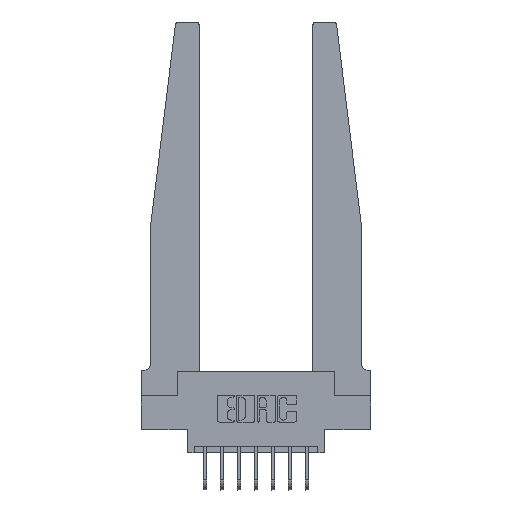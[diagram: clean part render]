
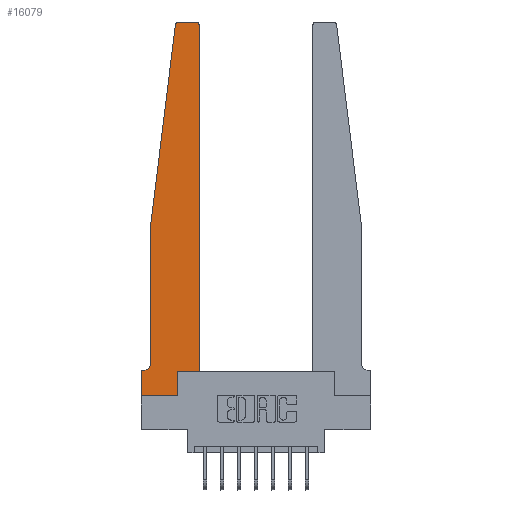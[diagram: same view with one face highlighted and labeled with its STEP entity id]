
A CAD part, top view. The second image highlights one B-rep face of the part: STEP entity #16079.
In plain terms, the highlighted planar face has unit normal (0, 0, 1).
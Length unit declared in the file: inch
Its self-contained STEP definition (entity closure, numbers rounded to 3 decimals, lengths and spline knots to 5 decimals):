
#207 = DIRECTION ( 'NONE',  ( -1., 0., 0. ) ) ;
#374 = ORIENTED_EDGE ( 'NONE', *, *, #4629, .T. ) ;
#394 = CARTESIAN_POINT ( 'NONE',  ( 0.425, 2.72, 0.37 ) ) ;
#516 = VECTOR ( 'NONE', #6131, 39.37008 ) ;
#575 = DIRECTION ( 'NONE',  ( 0., 0., 1. ) ) ;
#1018 = AXIS2_PLACEMENT_3D ( 'NONE', #13796, #10324, #2430 ) ;
#1557 = CARTESIAN_POINT ( 'NONE',  ( 0.425, 0.18, 0.37 ) ) ;
#1692 = EDGE_LOOP ( 'NONE', ( #10628, #9518, #12630, #6808, #10252, #374, #15915, #11730, #1996, #14589, #9808, #15762 ) ) ;
#1775 = AXIS2_PLACEMENT_3D ( 'NONE', #13913, #6101, #12507 ) ;
#1996 = ORIENTED_EDGE ( 'NONE', *, *, #5262, .T. ) ;
#2236 = CARTESIAN_POINT ( 'NONE',  ( 0.065, 1.25, 0.37 ) ) ;
#2331 = VECTOR ( 'NONE', #15895, 39.37008 ) ;
#2387 = VERTEX_POINT ( 'NONE', #10439 ) ;
#2430 = DIRECTION ( 'NONE',  ( 1., 0., 0. ) ) ;
#2669 = VECTOR ( 'NONE', #15243, 39.37008 ) ;
#2709 = VERTEX_POINT ( 'NONE', #15512 ) ;
#2909 = VECTOR ( 'NONE', #5039, 39.37008 ) ;
#3059 = EDGE_CURVE ( 'NONE', #3955, #15837, #10236, .T. ) ;
#3097 = EDGE_CURVE ( 'NONE', #10331, #5395, #7679, .T. ) ;
#3250 = CARTESIAN_POINT ( 'NONE',  ( 0.2605, 0., 0.37 ) ) ;
#3289 = VERTEX_POINT ( 'NONE', #9581 ) ;
#3299 = VERTEX_POINT ( 'NONE', #7547 ) ;
#3534 = FACE_OUTER_BOUND ( 'NONE', #1692, .T. ) ;
#3955 = VERTEX_POINT ( 'NONE', #16343 ) ;
#4003 = DIRECTION ( 'NONE',  ( 0., 1., 0. ) ) ;
#4544 = DIRECTION ( 'NONE',  ( 1., 0., 0. ) ) ;
#4629 = EDGE_CURVE ( 'NONE', #6245, #13054, #5420, .T. ) ;
#5039 = DIRECTION ( 'NONE',  ( 0., -1., 0. ) ) ;
#5262 = EDGE_CURVE ( 'NONE', #5395, #3299, #6387, .T. ) ;
#5395 = VERTEX_POINT ( 'NONE', #3250 ) ;
#5420 = LINE ( 'NONE', #14393, #2331 ) ;
#5678 = EDGE_CURVE ( 'NONE', #9020, #11882, #6043, .T. ) ;
#6015 = PLANE ( 'NONE',  #1775 ) ;
#6043 = CIRCLE ( 'NONE', #1018, 0.03 ) ;
#6101 = DIRECTION ( 'NONE',  ( 0., 0., 1. ) ) ;
#6131 = DIRECTION ( 'NONE',  ( 1., 0., 0. ) ) ;
#6245 = VERTEX_POINT ( 'NONE', #15722 ) ;
#6387 = LINE ( 'NONE', #15620, #8412 ) ;
#6808 = ORIENTED_EDGE ( 'NONE', *, *, #14761, .T. ) ;
#7057 = CARTESIAN_POINT ( 'NONE',  ( 0., 0., 0.37 ) ) ;
#7487 = EDGE_CURVE ( 'NONE', #13054, #10331, #11346, .T. ) ;
#7516 = CARTESIAN_POINT ( 'NONE',  ( 0., 0., 0.37 ) ) ;
#7547 = CARTESIAN_POINT ( 'NONE',  ( 0.2605, 0.18, 0.37 ) ) ;
#7679 = LINE ( 'NONE', #12775, #8087 ) ;
#7889 = LINE ( 'NONE', #8891, #11314 ) ;
#8087 = VECTOR ( 'NONE', #12926, 39.37008 ) ;
#8284 = CARTESIAN_POINT ( 'NONE',  ( 0., 0.1875, 0.37 ) ) ;
#8346 = CARTESIAN_POINT ( 'NONE',  ( 0.015, 0.2375, 0.37 ) ) ;
#8412 = VECTOR ( 'NONE', #4003, 39.37008 ) ;
#8523 = DIRECTION ( 'NONE',  ( 0., 0., -1. ) ) ;
#8667 = EDGE_CURVE ( 'NONE', #3299, #3955, #11277, .T. ) ;
#8891 = CARTESIAN_POINT ( 'NONE',  ( 0.25, 2.75, 0.37 ) ) ;
#9020 = VERTEX_POINT ( 'NONE', #11331 ) ;
#9503 = CARTESIAN_POINT ( 'NONE',  ( 0.395, 2.72, 0.37 ) ) ;
#9518 = ORIENTED_EDGE ( 'NONE', *, *, #5678, .T. ) ;
#9581 = CARTESIAN_POINT ( 'NONE',  ( 0.065, 0.2375, 0.37 ) ) ;
#9679 = DIRECTION ( 'NONE',  ( -1., 0., 0. ) ) ;
#9808 = ORIENTED_EDGE ( 'NONE', *, *, #3059, .T. ) ;
#10236 = LINE ( 'NONE', #1557, #16086 ) ;
#10252 = ORIENTED_EDGE ( 'NONE', *, *, #12363, .T. ) ;
#10324 = DIRECTION ( 'NONE',  ( 0., 0., 1. ) ) ;
#10331 = VERTEX_POINT ( 'NONE', #7057 ) ;
#10436 = CARTESIAN_POINT ( 'NONE',  ( 0.24675, 2.72367, 0.37 ) ) ;
#10439 = CARTESIAN_POINT ( 'NONE',  ( 0.395, 2.75, 0.37 ) ) ;
#10628 = ORIENTED_EDGE ( 'NONE', *, *, #16198, .T. ) ;
#11277 = LINE ( 'NONE', #16347, #516 ) ;
#11314 = VECTOR ( 'NONE', #207, 39.37008 ) ;
#11331 = CARTESIAN_POINT ( 'NONE',  ( 0.27653, 2.75, 0.37 ) ) ;
#11346 = LINE ( 'NONE', #7516, #2909 ) ;
#11730 = ORIENTED_EDGE ( 'NONE', *, *, #3097, .T. ) ;
#11882 = VERTEX_POINT ( 'NONE', #10436 ) ;
#12200 = CIRCLE ( 'NONE', #15642, 0.05 ) ;
#12363 = EDGE_CURVE ( 'NONE', #3289, #6245, #12200, .T. ) ;
#12507 = DIRECTION ( 'NONE',  ( 1., 0., 0. ) ) ;
#12630 = ORIENTED_EDGE ( 'NONE', *, *, #15260, .T. ) ;
#12775 = CARTESIAN_POINT ( 'NONE',  ( 0., 0., 0.37 ) ) ;
#12926 = DIRECTION ( 'NONE',  ( 1., 0., 0. ) ) ;
#13010 = VECTOR ( 'NONE', #14463, 39.37008 ) ;
#13054 = VERTEX_POINT ( 'NONE', #8284 ) ;
#13272 = AXIS2_PLACEMENT_3D ( 'NONE', #9503, #575, #4544 ) ;
#13605 = LINE ( 'NONE', #2236, #2669 ) ;
#13796 = CARTESIAN_POINT ( 'NONE',  ( 0.27653, 2.72, 0.37 ) ) ;
#13801 = CIRCLE ( 'NONE', #13272, 0.03 ) ;
#13913 = CARTESIAN_POINT ( 'NONE',  ( 0., 0.1875, 0.37 ) ) ;
#14384 = LINE ( 'NONE', #15547, #13010 ) ;
#14393 = CARTESIAN_POINT ( 'NONE',  ( 0.065, 0.1875, 0.37 ) ) ;
#14463 = DIRECTION ( 'NONE',  ( -0.122, -0.992, 0. ) ) ;
#14542 = EDGE_CURVE ( 'NONE', #15837, #2387, #13801, .T. ) ;
#14589 = ORIENTED_EDGE ( 'NONE', *, *, #8667, .T. ) ;
#14761 = EDGE_CURVE ( 'NONE', #2709, #3289, #13605, .T. ) ;
#15243 = DIRECTION ( 'NONE',  ( 0., -1., 0. ) ) ;
#15249 = DIRECTION ( 'NONE',  ( 0., 1., 0. ) ) ;
#15260 = EDGE_CURVE ( 'NONE', #11882, #2709, #14384, .T. ) ;
#15512 = CARTESIAN_POINT ( 'NONE',  ( 0.065, 1.25, 0.37 ) ) ;
#15547 = CARTESIAN_POINT ( 'NONE',  ( 0.065, 1.25, 0.37 ) ) ;
#15620 = CARTESIAN_POINT ( 'NONE',  ( 0.2605, 0.18, 0.37 ) ) ;
#15642 = AXIS2_PLACEMENT_3D ( 'NONE', #8346, #8523, #9679 ) ;
#15722 = CARTESIAN_POINT ( 'NONE',  ( 0.015, 0.1875, 0.37 ) ) ;
#15762 = ORIENTED_EDGE ( 'NONE', *, *, #14542, .T. ) ;
#15837 = VERTEX_POINT ( 'NONE', #394 ) ;
#15895 = DIRECTION ( 'NONE',  ( -1., 0., 0. ) ) ;
#15915 = ORIENTED_EDGE ( 'NONE', *, *, #7487, .T. ) ;
#16079 = ADVANCED_FACE ( 'NONE', ( #3534 ), #6015, .T. ) ;
#16086 = VECTOR ( 'NONE', #15249, 39.37008 ) ;
#16198 = EDGE_CURVE ( 'NONE', #2387, #9020, #7889, .T. ) ;
#16343 = CARTESIAN_POINT ( 'NONE',  ( 0.425, 0.18, 0.37 ) ) ;
#16347 = CARTESIAN_POINT ( 'NONE',  ( 0.425, 0.18, 0.37 ) ) ;
